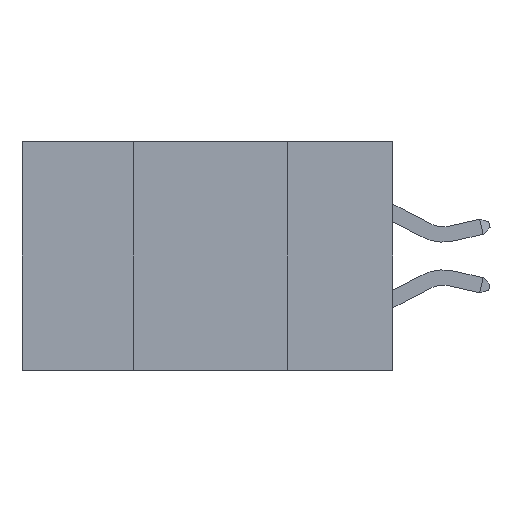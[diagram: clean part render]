
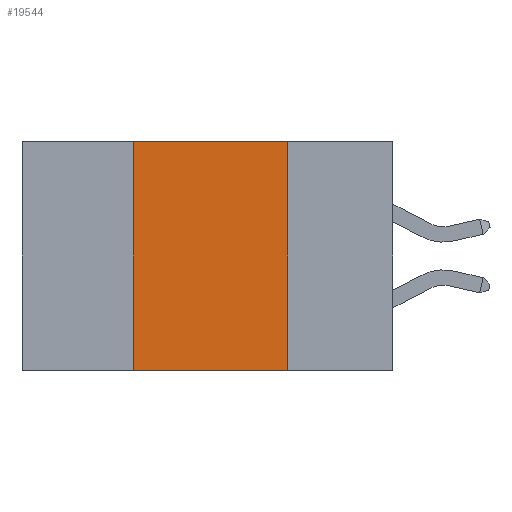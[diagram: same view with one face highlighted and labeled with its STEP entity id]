
A CAD part, left-side view. The second image highlights one B-rep face of the part: STEP entity #19544.
In plain terms, the highlighted planar face has unit normal (-1, 0, 0).
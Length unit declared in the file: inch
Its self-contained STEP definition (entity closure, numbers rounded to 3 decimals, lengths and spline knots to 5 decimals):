
#48 = EDGE_CURVE ( 'NONE', #6443, #12359, #4952, .T. ) ;
#74 = LINE ( 'NONE', #2937, #10891 ) ;
#321 = CARTESIAN_POINT ( 'NONE',  ( 0., 0.42, 0. ) ) ;
#2937 = CARTESIAN_POINT ( 'NONE',  ( 0., 0.6, 0. ) ) ;
#3269 = ORIENTED_EDGE ( 'NONE', *, *, #20310, .F. ) ;
#4006 = CARTESIAN_POINT ( 'NONE',  ( 0., 0.42, 0. ) ) ;
#4952 = LINE ( 'NONE', #18341, #23771 ) ;
#5103 = PLANE ( 'NONE',  #9793 ) ;
#5331 = DIRECTION ( 'NONE',  ( 0., 0., -1. ) ) ;
#5376 = VERTEX_POINT ( 'NONE', #4006 ) ;
#6039 = ORIENTED_EDGE ( 'NONE', *, *, #12154, .F. ) ;
#6443 = VERTEX_POINT ( 'NONE', #18991 ) ;
#7094 = LINE ( 'NONE', #13369, #15468 ) ;
#7461 = DIRECTION ( 'NONE',  ( 0., 0., -1. ) ) ;
#8554 = DIRECTION ( 'NONE',  ( 0., -1., 0. ) ) ;
#8852 = EDGE_LOOP ( 'NONE', ( #3269, #20726, #6039, #11813 ) ) ;
#9220 = DIRECTION ( 'NONE',  ( 1., 0., 0. ) ) ;
#9793 = AXIS2_PLACEMENT_3D ( 'NONE', #12830, #9220, #7461 ) ;
#10891 = VECTOR ( 'NONE', #8554, 39.37008 ) ;
#11813 = ORIENTED_EDGE ( 'NONE', *, *, #48, .T. ) ;
#11909 = DIRECTION ( 'NONE',  ( 0., 0., 1. ) ) ;
#12154 = EDGE_CURVE ( 'NONE', #6443, #5376, #22932, .T. ) ;
#12359 = VERTEX_POINT ( 'NONE', #20224 ) ;
#12830 = CARTESIAN_POINT ( 'NONE',  ( 0., 0.6, 0. ) ) ;
#13369 = CARTESIAN_POINT ( 'NONE',  ( 0., 0.17, 0. ) ) ;
#14845 = DIRECTION ( 'NONE',  ( 0., -1., 0. ) ) ;
#15468 = VECTOR ( 'NONE', #5331, 39.37008 ) ;
#15782 = CARTESIAN_POINT ( 'NONE',  ( 0., 0.17, 0. ) ) ;
#16979 = VECTOR ( 'NONE', #11909, 39.37008 ) ;
#18341 = CARTESIAN_POINT ( 'NONE',  ( 0., 0.6, -0.37 ) ) ;
#18767 = FACE_OUTER_BOUND ( 'NONE', #8852, .T. ) ;
#18991 = CARTESIAN_POINT ( 'NONE',  ( 0., 0.42, -0.37 ) ) ;
#19544 = ADVANCED_FACE ( 'NONE', ( #18767 ), #5103, .F. ) ;
#20224 = CARTESIAN_POINT ( 'NONE',  ( 0., 0.17, -0.37 ) ) ;
#20310 = EDGE_CURVE ( 'NONE', #24670, #12359, #7094, .T. ) ;
#20726 = ORIENTED_EDGE ( 'NONE', *, *, #22429, .F. ) ;
#22429 = EDGE_CURVE ( 'NONE', #5376, #24670, #74, .T. ) ;
#22932 = LINE ( 'NONE', #321, #16979 ) ;
#23771 = VECTOR ( 'NONE', #14845, 39.37008 ) ;
#24670 = VERTEX_POINT ( 'NONE', #15782 ) ;
